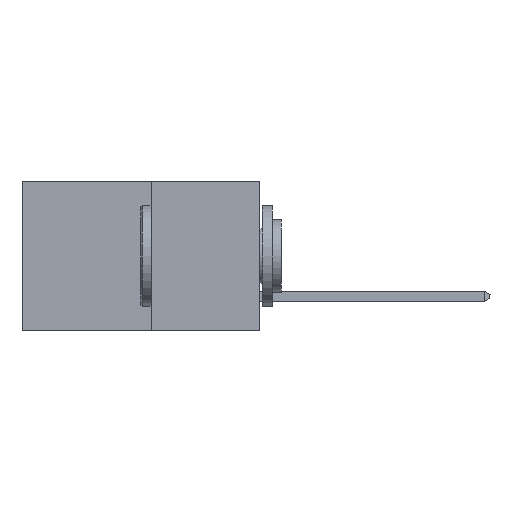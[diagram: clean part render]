
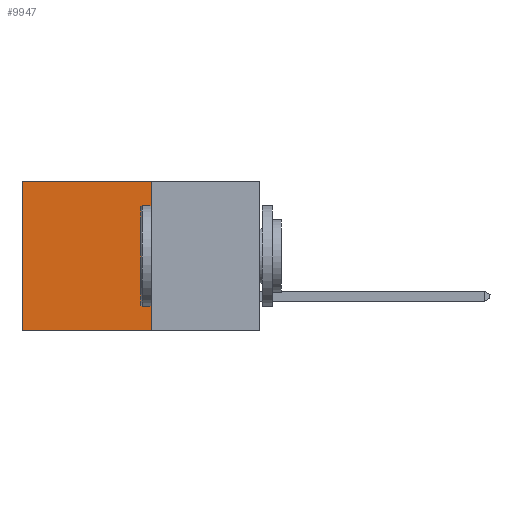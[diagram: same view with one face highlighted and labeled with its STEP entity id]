
A CAD part, left-side view. The second image highlights one B-rep face of the part: STEP entity #9947.
In plain terms, the highlighted planar face has unit normal (-1, 0, 0).
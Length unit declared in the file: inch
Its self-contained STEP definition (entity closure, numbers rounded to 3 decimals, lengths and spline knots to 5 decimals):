
#180 = CARTESIAN_POINT ( 'NONE',  ( 0.277, 0.27, -0.37 ) ) ;
#209 = CARTESIAN_POINT ( 'NONE',  ( 0.277, 0.27, 0. ) ) ;
#534 = CARTESIAN_POINT ( 'NONE',  ( 0.277, 0.59, 0. ) ) ;
#571 = ORIENTED_EDGE ( 'NONE', *, *, #6670, .T. ) ;
#824 = LINE ( 'NONE', #4973, #4902 ) ;
#853 = VECTOR ( 'NONE', #3721, 39.37008 ) ;
#869 = PLANE ( 'NONE',  #7895 ) ;
#1112 = LINE ( 'NONE', #7831, #853 ) ;
#1352 = LINE ( 'NONE', #180, #9904 ) ;
#1814 = EDGE_LOOP ( 'NONE', ( #571, #10514, #8304, #5848 ) ) ;
#2052 = VERTEX_POINT ( 'NONE', #8057 ) ;
#2776 = DIRECTION ( 'NONE',  ( 0., 1., 0. ) ) ;
#2819 = EDGE_CURVE ( 'NONE', #7228, #2052, #1112, .T. ) ;
#3721 = DIRECTION ( 'NONE',  ( 0., 0., -1. ) ) ;
#4362 = DIRECTION ( 'NONE',  ( 1., 0., 0. ) ) ;
#4800 = VECTOR ( 'NONE', #5620, 39.37008 ) ;
#4898 = DIRECTION ( 'NONE',  ( 0., 0., -1. ) ) ;
#4902 = VECTOR ( 'NONE', #4898, 39.37008 ) ;
#4973 = CARTESIAN_POINT ( 'NONE',  ( 0.277, 0.59, -0.37 ) ) ;
#5620 = DIRECTION ( 'NONE',  ( 0., 1., 0. ) ) ;
#5662 = VERTEX_POINT ( 'NONE', #10320 ) ;
#5848 = ORIENTED_EDGE ( 'NONE', *, *, #10255, .T. ) ;
#6670 = EDGE_CURVE ( 'NONE', #7770, #5662, #824, .T. ) ;
#7018 = EDGE_CURVE ( 'NONE', #2052, #5662, #1352, .T. ) ;
#7057 = LINE ( 'NONE', #8084, #4800 ) ;
#7228 = VERTEX_POINT ( 'NONE', #209 ) ;
#7770 = VERTEX_POINT ( 'NONE', #534 ) ;
#7831 = CARTESIAN_POINT ( 'NONE',  ( 0.277, 0.27, -0.37 ) ) ;
#7895 = AXIS2_PLACEMENT_3D ( 'NONE', #9269, #4362, #9994 ) ;
#8057 = CARTESIAN_POINT ( 'NONE',  ( 0.277, 0.27, -0.37 ) ) ;
#8084 = CARTESIAN_POINT ( 'NONE',  ( 0.277, 0.27, 0. ) ) ;
#8195 = FACE_OUTER_BOUND ( 'NONE', #1814, .T. ) ;
#8304 = ORIENTED_EDGE ( 'NONE', *, *, #2819, .F. ) ;
#9269 = CARTESIAN_POINT ( 'NONE',  ( 0.277, 0.27, -0.37 ) ) ;
#9904 = VECTOR ( 'NONE', #2776, 39.37008 ) ;
#9947 = ADVANCED_FACE ( 'NONE', ( #8195 ), #869, .F. ) ;
#9994 = DIRECTION ( 'NONE',  ( 0., 0., -1. ) ) ;
#10255 = EDGE_CURVE ( 'NONE', #7228, #7770, #7057, .T. ) ;
#10320 = CARTESIAN_POINT ( 'NONE',  ( 0.277, 0.59, -0.37 ) ) ;
#10514 = ORIENTED_EDGE ( 'NONE', *, *, #7018, .F. ) ;
